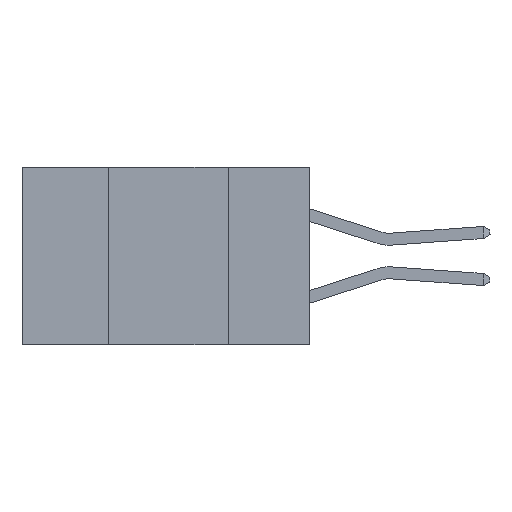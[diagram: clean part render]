
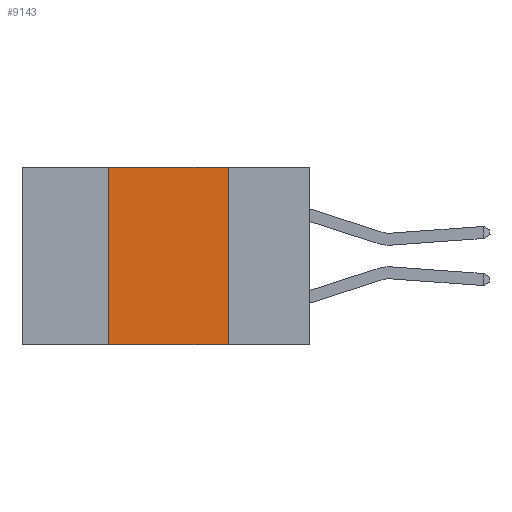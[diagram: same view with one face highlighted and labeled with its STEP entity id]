
A CAD part, left-side view. The second image highlights one B-rep face of the part: STEP entity #9143.
In plain terms, the highlighted planar face has unit normal (-1, 0, 0).
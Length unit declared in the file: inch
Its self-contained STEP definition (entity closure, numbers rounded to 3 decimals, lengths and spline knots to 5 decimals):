
#283 = CARTESIAN_POINT ( 'NONE',  ( 0., 0.6, 0. ) ) ;
#352 = CARTESIAN_POINT ( 'NONE',  ( 0., 0.6, -0.37 ) ) ;
#2789 = CARTESIAN_POINT ( 'NONE',  ( 0., 0.17, -0.37 ) ) ;
#3870 = ORIENTED_EDGE ( 'NONE', *, *, #15081, .T. ) ;
#4056 = EDGE_LOOP ( 'NONE', ( #15787, #7206, #16594, #3870 ) ) ;
#4538 = EDGE_CURVE ( 'NONE', #19653, #19471, #13221, .T. ) ;
#4874 = DIRECTION ( 'NONE',  ( 0., 0., -1. ) ) ;
#5195 = DIRECTION ( 'NONE',  ( 0., -1., 0. ) ) ;
#6070 = VERTEX_POINT ( 'NONE', #2789 ) ;
#6551 = LINE ( 'NONE', #12934, #9005 ) ;
#6556 = VERTEX_POINT ( 'NONE', #12119 ) ;
#6714 = DIRECTION ( 'NONE',  ( 1., 0., 0. ) ) ;
#7046 = CARTESIAN_POINT ( 'NONE',  ( 0., 0.6, 0. ) ) ;
#7206 = ORIENTED_EDGE ( 'NONE', *, *, #4538, .F. ) ;
#7698 = CARTESIAN_POINT ( 'NONE',  ( 0., 0.42, -0.37 ) ) ;
#7950 = AXIS2_PLACEMENT_3D ( 'NONE', #283, #6714, #13100 ) ;
#8309 = CARTESIAN_POINT ( 'NONE',  ( 0., 0.17, 0. ) ) ;
#9005 = VECTOR ( 'NONE', #4874, 39.37008 ) ;
#9143 = ADVANCED_FACE ( 'NONE', ( #13197 ), #14472, .F. ) ;
#10829 = LINE ( 'NONE', #7698, #12764 ) ;
#12119 = CARTESIAN_POINT ( 'NONE',  ( 0., 0.42, -0.37 ) ) ;
#12261 = VECTOR ( 'NONE', #18243, 39.37008 ) ;
#12764 = VECTOR ( 'NONE', #17305, 39.37008 ) ;
#12934 = CARTESIAN_POINT ( 'NONE',  ( 0., 0.17, -0.37 ) ) ;
#13100 = DIRECTION ( 'NONE',  ( 0., 0., -1. ) ) ;
#13197 = FACE_OUTER_BOUND ( 'NONE', #4056, .T. ) ;
#13221 = LINE ( 'NONE', #7046, #12261 ) ;
#13450 = EDGE_CURVE ( 'NONE', #19471, #6070, #6551, .T. ) ;
#14472 = PLANE ( 'NONE',  #7950 ) ;
#15081 = EDGE_CURVE ( 'NONE', #6556, #6070, #19550, .T. ) ;
#15402 = EDGE_CURVE ( 'NONE', #6556, #19653, #10829, .T. ) ;
#15787 = ORIENTED_EDGE ( 'NONE', *, *, #13450, .F. ) ;
#16594 = ORIENTED_EDGE ( 'NONE', *, *, #15402, .F. ) ;
#17305 = DIRECTION ( 'NONE',  ( 0., 0., 1. ) ) ;
#18243 = DIRECTION ( 'NONE',  ( 0., -1., 0. ) ) ;
#18248 = CARTESIAN_POINT ( 'NONE',  ( 0., 0.42, 0. ) ) ;
#18756 = VECTOR ( 'NONE', #5195, 39.37008 ) ;
#19471 = VERTEX_POINT ( 'NONE', #8309 ) ;
#19550 = LINE ( 'NONE', #352, #18756 ) ;
#19653 = VERTEX_POINT ( 'NONE', #18248 ) ;
